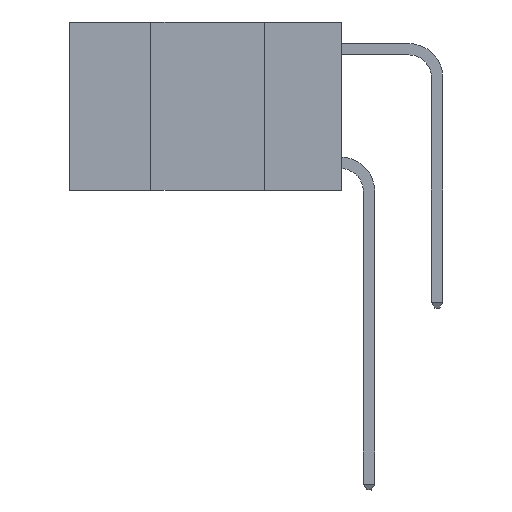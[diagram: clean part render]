
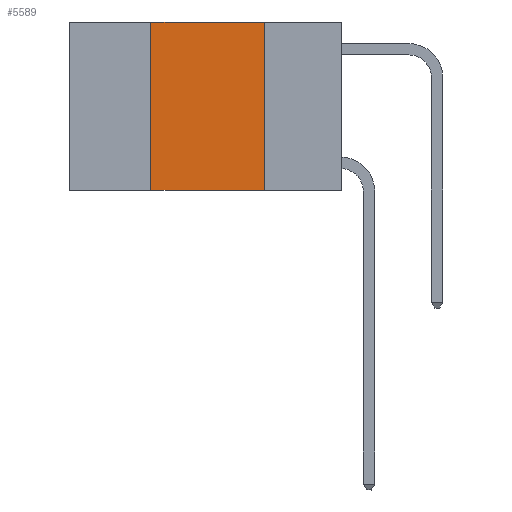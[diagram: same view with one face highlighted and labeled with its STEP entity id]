
A CAD part, left-side view. The second image highlights one B-rep face of the part: STEP entity #5589.
In plain terms, the highlighted planar face has unit normal (-1, 0, 0).
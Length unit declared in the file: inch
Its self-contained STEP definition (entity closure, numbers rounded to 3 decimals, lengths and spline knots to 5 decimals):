
#1642 = LINE ( 'NONE', #6496, #7292 ) ;
#1745 = AXIS2_PLACEMENT_3D ( 'NONE', #9112, #4627, #12607 ) ;
#2250 = CARTESIAN_POINT ( 'NONE',  ( 0., 0.42, 0. ) ) ;
#2384 = VECTOR ( 'NONE', #10706, 39.37008 ) ;
#2579 = EDGE_CURVE ( 'NONE', #7320, #9248, #10356, .T. ) ;
#2736 = ORIENTED_EDGE ( 'NONE', *, *, #2579, .F. ) ;
#2772 = EDGE_LOOP ( 'NONE', ( #2736, #8711, #11803, #12515 ) ) ;
#3088 = EDGE_CURVE ( 'NONE', #10183, #9248, #9249, .T. ) ;
#3312 = CARTESIAN_POINT ( 'NONE',  ( 0., 0.17, 0. ) ) ;
#3921 = CARTESIAN_POINT ( 'NONE',  ( 0., 0.6, 0. ) ) ;
#4627 = DIRECTION ( 'NONE',  ( 1., 0., 0. ) ) ;
#5586 = DIRECTION ( 'NONE',  ( 0., 0., -1. ) ) ;
#5589 = ADVANCED_FACE ( 'NONE', ( #5658 ), #9068, .F. ) ;
#5658 = FACE_OUTER_BOUND ( 'NONE', #2772, .T. ) ;
#6069 = VERTEX_POINT ( 'NONE', #2250 ) ;
#6496 = CARTESIAN_POINT ( 'NONE',  ( 0., 0.42, 0. ) ) ;
#6989 = VECTOR ( 'NONE', #5586, 39.37008 ) ;
#7292 = VECTOR ( 'NONE', #7625, 39.37008 ) ;
#7320 = VERTEX_POINT ( 'NONE', #3312 ) ;
#7625 = DIRECTION ( 'NONE',  ( 0., 0., 1. ) ) ;
#7681 = LINE ( 'NONE', #3921, #2384 ) ;
#8711 = ORIENTED_EDGE ( 'NONE', *, *, #11900, .F. ) ;
#9068 = PLANE ( 'NONE',  #1745 ) ;
#9112 = CARTESIAN_POINT ( 'NONE',  ( 0., 0.6, 0. ) ) ;
#9248 = VERTEX_POINT ( 'NONE', #10899 ) ;
#9249 = LINE ( 'NONE', #9800, #12705 ) ;
#9800 = CARTESIAN_POINT ( 'NONE',  ( 0., 0.6, -0.37 ) ) ;
#10183 = VERTEX_POINT ( 'NONE', #10213 ) ;
#10213 = CARTESIAN_POINT ( 'NONE',  ( 0., 0.42, -0.37 ) ) ;
#10356 = LINE ( 'NONE', #14665, #6989 ) ;
#10706 = DIRECTION ( 'NONE',  ( 0., -1., 0. ) ) ;
#10899 = CARTESIAN_POINT ( 'NONE',  ( 0., 0.17, -0.37 ) ) ;
#10979 = DIRECTION ( 'NONE',  ( 0., -1., 0. ) ) ;
#11803 = ORIENTED_EDGE ( 'NONE', *, *, #13249, .F. ) ;
#11900 = EDGE_CURVE ( 'NONE', #6069, #7320, #7681, .T. ) ;
#12515 = ORIENTED_EDGE ( 'NONE', *, *, #3088, .T. ) ;
#12607 = DIRECTION ( 'NONE',  ( 0., 0., -1. ) ) ;
#12705 = VECTOR ( 'NONE', #10979, 39.37008 ) ;
#13249 = EDGE_CURVE ( 'NONE', #10183, #6069, #1642, .T. ) ;
#14665 = CARTESIAN_POINT ( 'NONE',  ( 0., 0.17, 0. ) ) ;
